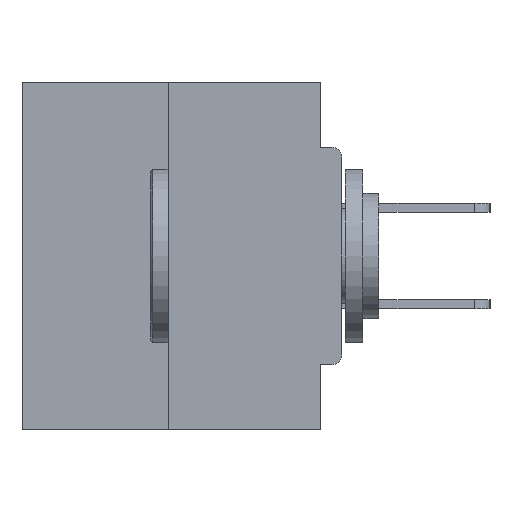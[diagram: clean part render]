
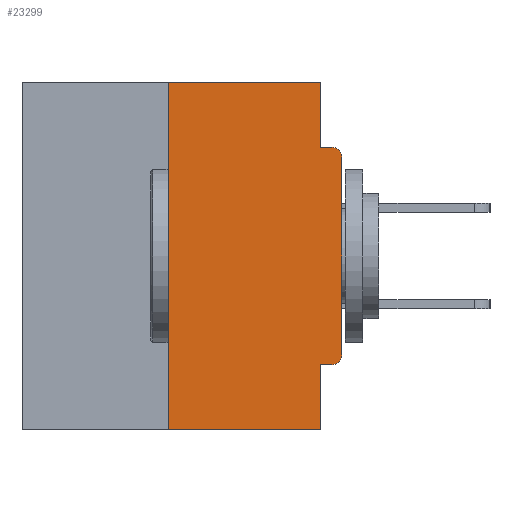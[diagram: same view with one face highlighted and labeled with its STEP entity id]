
A CAD part, left-side view. The second image highlights one B-rep face of the part: STEP entity #23299.
In plain terms, the highlighted planar face has unit normal (-1, 0, 0).
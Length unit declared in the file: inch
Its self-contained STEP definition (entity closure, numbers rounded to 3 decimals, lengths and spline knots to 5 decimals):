
#1725 = CARTESIAN_POINT ( 'NONE',  ( 0., 0.25, -0.5 ) ) ;
#2457 = VERTEX_POINT ( 'NONE', #6694 ) ;
#3077 = EDGE_CURVE ( 'NONE', #6245, #24904, #23617, .T. ) ;
#3115 = CARTESIAN_POINT ( 'NONE',  ( 0., 0.015, -0.0935 ) ) ;
#3275 = CIRCLE ( 'NONE', #17649, 0.015 ) ;
#3591 = VECTOR ( 'NONE', #30514, 39.37008 ) ;
#4258 = EDGE_CURVE ( 'NONE', #9138, #26541, #29148, .T. ) ;
#4344 = DIRECTION ( 'NONE',  ( 1., 0., 0. ) ) ;
#4457 = CARTESIAN_POINT ( 'NONE',  ( 0., 0.031, -0.5 ) ) ;
#5285 = EDGE_LOOP ( 'NONE', ( #6014, #25553, #20990, #14930, #17990, #8653, #27628, #29158, #8685, #32624 ) ) ;
#6014 = ORIENTED_EDGE ( 'NONE', *, *, #4258, .F. ) ;
#6228 = VERTEX_POINT ( 'NONE', #11508 ) ;
#6245 = VERTEX_POINT ( 'NONE', #19176 ) ;
#6392 = CARTESIAN_POINT ( 'NONE',  ( 0., 0.015, -0.1085 ) ) ;
#6694 = CARTESIAN_POINT ( 'NONE',  ( 0., 0.031, -0.4065 ) ) ;
#6804 = AXIS2_PLACEMENT_3D ( 'NONE', #14747, #32536, #17343 ) ;
#6888 = DIRECTION ( 'NONE',  ( 0., 0., -1. ) ) ;
#7208 = VERTEX_POINT ( 'NONE', #1725 ) ;
#7419 = CARTESIAN_POINT ( 'NONE',  ( 0., 0., -0.0935 ) ) ;
#7513 = CARTESIAN_POINT ( 'NONE',  ( 0., 0.46, 0. ) ) ;
#7720 = VECTOR ( 'NONE', #16907, 39.37008 ) ;
#8653 = ORIENTED_EDGE ( 'NONE', *, *, #18216, .T. ) ;
#8685 = ORIENTED_EDGE ( 'NONE', *, *, #3077, .F. ) ;
#8971 = DIRECTION ( 'NONE',  ( 0., 0., -1. ) ) ;
#9138 = VERTEX_POINT ( 'NONE', #22359 ) ;
#9240 = FACE_OUTER_BOUND ( 'NONE', #5285, .T. ) ;
#9503 = LINE ( 'NONE', #24530, #23020 ) ;
#9895 = LINE ( 'NONE', #4457, #10213 ) ;
#10213 = VECTOR ( 'NONE', #6888, 39.37008 ) ;
#10297 = CARTESIAN_POINT ( 'NONE',  ( 0., 0., -0.1085 ) ) ;
#11330 = AXIS2_PLACEMENT_3D ( 'NONE', #11992, #4344, #8971 ) ;
#11508 = CARTESIAN_POINT ( 'NONE',  ( 0., 0.031, -0.5 ) ) ;
#11553 = VERTEX_POINT ( 'NONE', #19684 ) ;
#11992 = CARTESIAN_POINT ( 'NONE',  ( 0., 0.46, 0. ) ) ;
#12640 = DIRECTION ( 'NONE',  ( 0., -1., 0. ) ) ;
#12747 = CARTESIAN_POINT ( 'NONE',  ( 0., 0., 0. ) ) ;
#14292 = EDGE_CURVE ( 'NONE', #7208, #6228, #32297, .T. ) ;
#14327 = CARTESIAN_POINT ( 'NONE',  ( 0., 0.25, 0. ) ) ;
#14479 = LINE ( 'NONE', #14327, #7720 ) ;
#14747 = CARTESIAN_POINT ( 'NONE',  ( 0., 0.015, -0.3915 ) ) ;
#14930 = ORIENTED_EDGE ( 'NONE', *, *, #30397, .F. ) ;
#15395 = LINE ( 'NONE', #20541, #18974 ) ;
#16907 = DIRECTION ( 'NONE',  ( 0., 0., 1. ) ) ;
#17202 = VECTOR ( 'NONE', #30712, 39.37008 ) ;
#17343 = DIRECTION ( 'NONE',  ( 0., 0., -1. ) ) ;
#17490 = LINE ( 'NONE', #12747, #3591 ) ;
#17649 = AXIS2_PLACEMENT_3D ( 'NONE', #6392, #18896, #23801 ) ;
#17658 = EDGE_CURVE ( 'NONE', #21923, #2457, #15395, .T. ) ;
#17990 = ORIENTED_EDGE ( 'NONE', *, *, #17658, .F. ) ;
#18216 = EDGE_CURVE ( 'NONE', #21923, #11553, #26279, .T. ) ;
#18896 = DIRECTION ( 'NONE',  ( -1., 0., 0. ) ) ;
#18974 = VECTOR ( 'NONE', #23101, 39.37008 ) ;
#19176 = CARTESIAN_POINT ( 'NONE',  ( 0., 0.031, -0.0935 ) ) ;
#19442 = CARTESIAN_POINT ( 'NONE',  ( 0., 0.015, -0.4065 ) ) ;
#19535 = PLANE ( 'NONE',  #11330 ) ;
#19684 = CARTESIAN_POINT ( 'NONE',  ( 0., 0., -0.3915 ) ) ;
#20541 = CARTESIAN_POINT ( 'NONE',  ( 0., 0., -0.4065 ) ) ;
#20990 = ORIENTED_EDGE ( 'NONE', *, *, #14292, .T. ) ;
#21037 = VERTEX_POINT ( 'NONE', #10297 ) ;
#21923 = VERTEX_POINT ( 'NONE', #19442 ) ;
#21977 = EDGE_CURVE ( 'NONE', #7208, #9138, #14479, .T. ) ;
#22206 = CARTESIAN_POINT ( 'NONE',  ( 0., 0.46, -0.5 ) ) ;
#22359 = CARTESIAN_POINT ( 'NONE',  ( 0., 0.25, 0. ) ) ;
#23020 = VECTOR ( 'NONE', #24426, 39.37008 ) ;
#23101 = DIRECTION ( 'NONE',  ( 0., 1., 0. ) ) ;
#23299 = ADVANCED_FACE ( 'NONE', ( #9240 ), #19535, .F. ) ;
#23617 = LINE ( 'NONE', #7419, #26852 ) ;
#23801 = DIRECTION ( 'NONE',  ( 0., 0., -1. ) ) ;
#24426 = DIRECTION ( 'NONE',  ( 0., 0., -1. ) ) ;
#24530 = CARTESIAN_POINT ( 'NONE',  ( 0., 0.031, 0. ) ) ;
#24904 = VERTEX_POINT ( 'NONE', #3115 ) ;
#25553 = ORIENTED_EDGE ( 'NONE', *, *, #21977, .F. ) ;
#26279 = CIRCLE ( 'NONE', #6804, 0.015 ) ;
#26541 = VERTEX_POINT ( 'NONE', #31327 ) ;
#26852 = VECTOR ( 'NONE', #12640, 39.37008 ) ;
#27044 = EDGE_CURVE ( 'NONE', #21037, #24904, #3275, .T. ) ;
#27628 = ORIENTED_EDGE ( 'NONE', *, *, #28372, .T. ) ;
#28372 = EDGE_CURVE ( 'NONE', #11553, #21037, #17490, .T. ) ;
#29148 = LINE ( 'NONE', #7513, #30329 ) ;
#29158 = ORIENTED_EDGE ( 'NONE', *, *, #27044, .T. ) ;
#29550 = EDGE_CURVE ( 'NONE', #26541, #6245, #9503, .T. ) ;
#30329 = VECTOR ( 'NONE', #32524, 39.37008 ) ;
#30397 = EDGE_CURVE ( 'NONE', #2457, #6228, #9895, .T. ) ;
#30514 = DIRECTION ( 'NONE',  ( 0., 0., 1. ) ) ;
#30712 = DIRECTION ( 'NONE',  ( 0., -1., 0. ) ) ;
#31327 = CARTESIAN_POINT ( 'NONE',  ( 0., 0.031, 0. ) ) ;
#32297 = LINE ( 'NONE', #22206, #17202 ) ;
#32524 = DIRECTION ( 'NONE',  ( 0., -1., 0. ) ) ;
#32536 = DIRECTION ( 'NONE',  ( -1., 0., 0. ) ) ;
#32624 = ORIENTED_EDGE ( 'NONE', *, *, #29550, .F. ) ;
